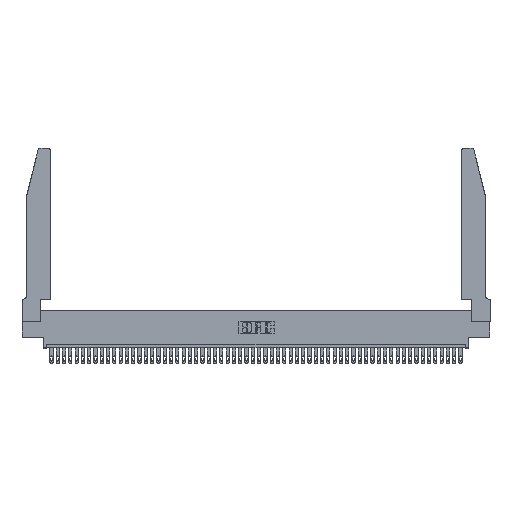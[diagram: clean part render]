
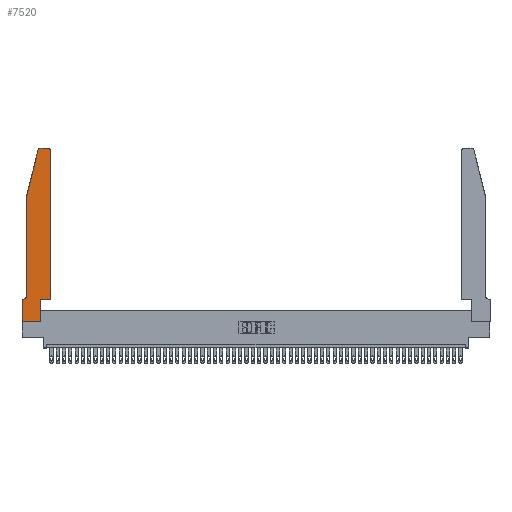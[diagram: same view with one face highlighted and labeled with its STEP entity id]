
A CAD part, top view. The second image highlights one B-rep face of the part: STEP entity #7520.
In plain terms, the highlighted planar face has unit normal (0, 0, 1).
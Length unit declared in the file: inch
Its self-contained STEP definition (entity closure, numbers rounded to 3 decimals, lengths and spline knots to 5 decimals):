
#1853 = EDGE_CURVE ( 'NONE', #36636, #12830, #11165, .T. ) ;
#1872 = VERTEX_POINT ( 'NONE', #31976 ) ;
#2034 = CARTESIAN_POINT ( 'NONE',  ( 0.0755, 2., 0.37 ) ) ;
#2103 = DIRECTION ( 'NONE',  ( 0., 0., 1. ) ) ;
#2186 = LINE ( 'NONE', #2663, #24386 ) ;
#2239 = CARTESIAN_POINT ( 'NONE',  ( 0.284, 2.75, 0.37 ) ) ;
#2508 = VECTOR ( 'NONE', #8464, 39.37008 ) ;
#2663 = CARTESIAN_POINT ( 'NONE',  ( 0.4505, 0.35, 0.37 ) ) ;
#3098 = ORIENTED_EDGE ( 'NONE', *, *, #40477, .T. ) ;
#4212 = ORIENTED_EDGE ( 'NONE', *, *, #38376, .T. ) ;
#4583 = EDGE_LOOP ( 'NONE', ( #20586, #10118, #7273, #41770, #4212, #20839, #31906, #6644, #23221, #3098, #16538, #17567 ) ) ;
#5100 = VECTOR ( 'NONE', #13816, 39.37008 ) ;
#5642 = LINE ( 'NONE', #41735, #16119 ) ;
#6068 = DIRECTION ( 'NONE',  ( 1., 0., 0. ) ) ;
#6318 = CARTESIAN_POINT ( 'NONE',  ( 0.4505, 2.72, 0.37 ) ) ;
#6431 = CIRCLE ( 'NONE', #38073, 0.03 ) ;
#6644 = ORIENTED_EDGE ( 'NONE', *, *, #48387, .T. ) ;
#7273 = ORIENTED_EDGE ( 'NONE', *, *, #46429, .T. ) ;
#7520 = ADVANCED_FACE ( 'NONE', ( #37700 ), #26928, .T. ) ;
#7747 = CARTESIAN_POINT ( 'NONE',  ( 0.25487, 2.72718, 0.37 ) ) ;
#8394 = CARTESIAN_POINT ( 'NONE',  ( 0.0055, 0.35, 0.37 ) ) ;
#8464 = DIRECTION ( 'NONE',  ( 0., 1., 0. ) ) ;
#8810 = VERTEX_POINT ( 'NONE', #6318 ) ;
#8886 = VECTOR ( 'NONE', #33803, 39.37008 ) ;
#9175 = CARTESIAN_POINT ( 'NONE',  ( 0., 0., 0.37 ) ) ;
#10118 = ORIENTED_EDGE ( 'NONE', *, *, #36833, .T. ) ;
#10686 = LINE ( 'NONE', #25690, #5100 ) ;
#10799 = LINE ( 'NONE', #44633, #34885 ) ;
#11165 = LINE ( 'NONE', #32463, #34640 ) ;
#12830 = VERTEX_POINT ( 'NONE', #2239 ) ;
#13816 = DIRECTION ( 'NONE',  ( 0., -1., 0. ) ) ;
#14507 = VERTEX_POINT ( 'NONE', #7747 ) ;
#14703 = DIRECTION ( 'NONE',  ( 1., 0., 0. ) ) ;
#16119 = VECTOR ( 'NONE', #25184, 39.37008 ) ;
#16151 = AXIS2_PLACEMENT_3D ( 'NONE', #45209, #2103, #6068 ) ;
#16538 = ORIENTED_EDGE ( 'NONE', *, *, #39131, .T. ) ;
#17567 = ORIENTED_EDGE ( 'NONE', *, *, #37927, .T. ) ;
#19155 = CARTESIAN_POINT ( 'NONE',  ( 0., 0.35, 0.37 ) ) ;
#20586 = ORIENTED_EDGE ( 'NONE', *, *, #1853, .T. ) ;
#20839 = ORIENTED_EDGE ( 'NONE', *, *, #44065, .T. ) ;
#21431 = AXIS2_PLACEMENT_3D ( 'NONE', #42876, #26880, #38897 ) ;
#23111 = CARTESIAN_POINT ( 'NONE',  ( 0.0755, 0.42, 0.37 ) ) ;
#23117 = DIRECTION ( 'NONE',  ( 0., 0., 1. ) ) ;
#23221 = ORIENTED_EDGE ( 'NONE', *, *, #26080, .T. ) ;
#23725 = VERTEX_POINT ( 'NONE', #35470 ) ;
#24256 = CARTESIAN_POINT ( 'NONE',  ( 0.4505, 0.35, 0.37 ) ) ;
#24386 = VECTOR ( 'NONE', #14703, 39.37008 ) ;
#25184 = DIRECTION ( 'NONE',  ( 0., -1., 0. ) ) ;
#25690 = CARTESIAN_POINT ( 'NONE',  ( 0., 0., 0.37 ) ) ;
#26080 = EDGE_CURVE ( 'NONE', #41842, #36224, #44403, .T. ) ;
#26880 = DIRECTION ( 'NONE',  ( 0., 0., -1. ) ) ;
#26896 = VERTEX_POINT ( 'NONE', #24256 ) ;
#26899 = VERTEX_POINT ( 'NONE', #8394 ) ;
#26928 = PLANE ( 'NONE',  #46418 ) ;
#27604 = CARTESIAN_POINT ( 'NONE',  ( 0.2865, 0.35, 0.37 ) ) ;
#27746 = EDGE_CURVE ( 'NONE', #23725, #30961, #10686, .T. ) ;
#27834 = EDGE_CURVE ( 'NONE', #1872, #39573, #5642, .T. ) ;
#28098 = CARTESIAN_POINT ( 'NONE',  ( 0.2865, 0.35, 0.37 ) ) ;
#28181 = CARTESIAN_POINT ( 'NONE',  ( 0.2865, 0., 0.37 ) ) ;
#28459 = LINE ( 'NONE', #9175, #49593 ) ;
#30961 = VERTEX_POINT ( 'NONE', #31866 ) ;
#31638 = DIRECTION ( 'NONE',  ( 0., 0., 1. ) ) ;
#31866 = CARTESIAN_POINT ( 'NONE',  ( 0., 0., 0.37 ) ) ;
#31906 = ORIENTED_EDGE ( 'NONE', *, *, #27746, .T. ) ;
#31976 = CARTESIAN_POINT ( 'NONE',  ( 0.0755, 2., 0.37 ) ) ;
#32416 = DIRECTION ( 'NONE',  ( -1., 0., 0. ) ) ;
#32463 = CARTESIAN_POINT ( 'NONE',  ( 0.2605, 2.75, 0.37 ) ) ;
#32649 = DIRECTION ( 'NONE',  ( -1., 0., 0. ) ) ;
#33160 = VECTOR ( 'NONE', #39332, 39.37008 ) ;
#33551 = CARTESIAN_POINT ( 'NONE',  ( 0.4205, 2.75, 0.37 ) ) ;
#33803 = DIRECTION ( 'NONE',  ( -0.239, -0.971, 0. ) ) ;
#34001 = LINE ( 'NONE', #47778, #2508 ) ;
#34640 = VECTOR ( 'NONE', #32649, 39.37008 ) ;
#34885 = VECTOR ( 'NONE', #32416, 39.37008 ) ;
#35470 = CARTESIAN_POINT ( 'NONE',  ( 0., 0.35, 0.37 ) ) ;
#35624 = DIRECTION ( 'NONE',  ( 1., 0., 0. ) ) ;
#36224 = VERTEX_POINT ( 'NONE', #27604 ) ;
#36636 = VERTEX_POINT ( 'NONE', #33551 ) ;
#36833 = EDGE_CURVE ( 'NONE', #12830, #14507, #6431, .T. ) ;
#36872 = DIRECTION ( 'NONE',  ( 1., 0., 0. ) ) ;
#37700 = FACE_OUTER_BOUND ( 'NONE', #4583, .T. ) ;
#37927 = EDGE_CURVE ( 'NONE', #8810, #36636, #47792, .T. ) ;
#38073 = AXIS2_PLACEMENT_3D ( 'NONE', #48253, #31638, #35624 ) ;
#38376 = EDGE_CURVE ( 'NONE', #39573, #26899, #47186, .T. ) ;
#38897 = DIRECTION ( 'NONE',  ( -1., 0., 0. ) ) ;
#39131 = EDGE_CURVE ( 'NONE', #26896, #8810, #34001, .T. ) ;
#39332 = DIRECTION ( 'NONE',  ( 0., 1., 0. ) ) ;
#39573 = VERTEX_POINT ( 'NONE', #23111 ) ;
#40477 = EDGE_CURVE ( 'NONE', #36224, #26896, #2186, .T. ) ;
#41158 = LINE ( 'NONE', #2034, #8886 ) ;
#41735 = CARTESIAN_POINT ( 'NONE',  ( 0.0755, 2., 0.37 ) ) ;
#41770 = ORIENTED_EDGE ( 'NONE', *, *, #27834, .T. ) ;
#41842 = VERTEX_POINT ( 'NONE', #28181 ) ;
#42876 = CARTESIAN_POINT ( 'NONE',  ( 0.0055, 0.42, 0.37 ) ) ;
#43102 = DIRECTION ( 'NONE',  ( 1., 0., 0. ) ) ;
#44065 = EDGE_CURVE ( 'NONE', #26899, #23725, #10799, .T. ) ;
#44403 = LINE ( 'NONE', #28098, #33160 ) ;
#44633 = CARTESIAN_POINT ( 'NONE',  ( 0.0755, 0.35, 0.37 ) ) ;
#45209 = CARTESIAN_POINT ( 'NONE',  ( 0.4205, 2.72, 0.37 ) ) ;
#46418 = AXIS2_PLACEMENT_3D ( 'NONE', #19155, #23117, #43102 ) ;
#46429 = EDGE_CURVE ( 'NONE', #14507, #1872, #41158, .T. ) ;
#47186 = CIRCLE ( 'NONE', #21431, 0.07 ) ;
#47778 = CARTESIAN_POINT ( 'NONE',  ( 0.4505, 0.35, 0.37 ) ) ;
#47792 = CIRCLE ( 'NONE', #16151, 0.03 ) ;
#48253 = CARTESIAN_POINT ( 'NONE',  ( 0.284, 2.72, 0.37 ) ) ;
#48387 = EDGE_CURVE ( 'NONE', #30961, #41842, #28459, .T. ) ;
#49593 = VECTOR ( 'NONE', #36872, 39.37008 ) ;
